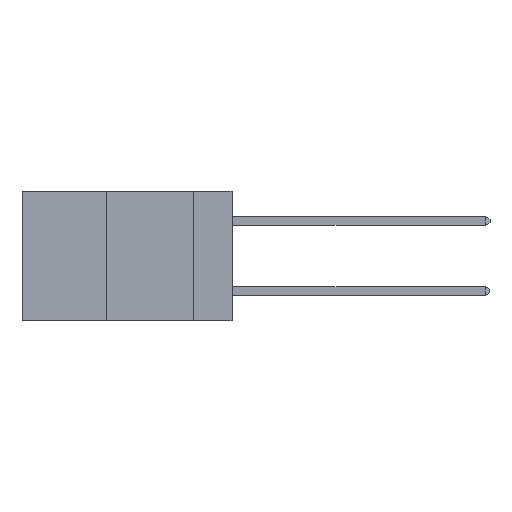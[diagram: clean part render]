
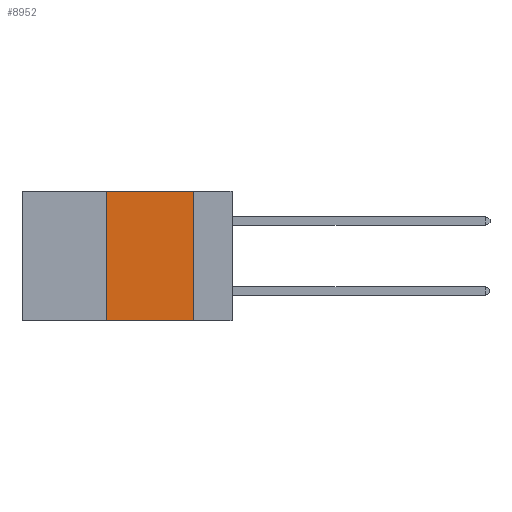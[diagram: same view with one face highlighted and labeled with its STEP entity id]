
A CAD part, left-side view. The second image highlights one B-rep face of the part: STEP entity #8952.
In plain terms, the highlighted planar face has unit normal (-1, 0, 0).
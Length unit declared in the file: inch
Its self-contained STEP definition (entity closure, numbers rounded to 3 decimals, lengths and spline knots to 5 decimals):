
#103 = LINE ( 'NONE', #3555, #1944 ) ;
#345 = ORIENTED_EDGE ( 'NONE', *, *, #6749, .T. ) ;
#522 = DIRECTION ( 'NONE',  ( 0., 0., -1. ) ) ;
#598 = LINE ( 'NONE', #9883, #2909 ) ;
#654 = VECTOR ( 'NONE', #4590, 39.37008 ) ;
#705 = CARTESIAN_POINT ( 'NONE',  ( 0., 0.6, -0.37 ) ) ;
#973 = CARTESIAN_POINT ( 'NONE',  ( 0., 0.36, -0.37 ) ) ;
#1944 = VECTOR ( 'NONE', #6691, 39.37008 ) ;
#2097 = LINE ( 'NONE', #9091, #6032 ) ;
#2643 = CARTESIAN_POINT ( 'NONE',  ( 0., 0.11, 0. ) ) ;
#2756 = PLANE ( 'NONE',  #9317 ) ;
#2809 = VERTEX_POINT ( 'NONE', #3524 ) ;
#2909 = VECTOR ( 'NONE', #5192, 39.37008 ) ;
#3524 = CARTESIAN_POINT ( 'NONE',  ( 0., 0.11, -0.37 ) ) ;
#3554 = CARTESIAN_POINT ( 'NONE',  ( 0., 0.6, 0. ) ) ;
#3555 = CARTESIAN_POINT ( 'NONE',  ( 0., 0.6, 0. ) ) ;
#3788 = ORIENTED_EDGE ( 'NONE', *, *, #3938, .F. ) ;
#3938 = EDGE_CURVE ( 'NONE', #5005, #7772, #103, .T. ) ;
#4338 = DIRECTION ( 'NONE',  ( 1., 0., 0. ) ) ;
#4590 = DIRECTION ( 'NONE',  ( 0., -1., 0. ) ) ;
#5005 = VERTEX_POINT ( 'NONE', #7924 ) ;
#5192 = DIRECTION ( 'NONE',  ( 0., 0., 1. ) ) ;
#5319 = EDGE_LOOP ( 'NONE', ( #7978, #3788, #7088, #345 ) ) ;
#5479 = FACE_OUTER_BOUND ( 'NONE', #5319, .T. ) ;
#6032 = VECTOR ( 'NONE', #522, 39.37008 ) ;
#6320 = VERTEX_POINT ( 'NONE', #973 ) ;
#6601 = EDGE_CURVE ( 'NONE', #7772, #2809, #2097, .T. ) ;
#6691 = DIRECTION ( 'NONE',  ( 0., -1., 0. ) ) ;
#6749 = EDGE_CURVE ( 'NONE', #6320, #2809, #6906, .T. ) ;
#6906 = LINE ( 'NONE', #705, #654 ) ;
#7088 = ORIENTED_EDGE ( 'NONE', *, *, #8997, .F. ) ;
#7772 = VERTEX_POINT ( 'NONE', #2643 ) ;
#7924 = CARTESIAN_POINT ( 'NONE',  ( 0., 0.36, 0. ) ) ;
#7978 = ORIENTED_EDGE ( 'NONE', *, *, #6601, .F. ) ;
#8952 = ADVANCED_FACE ( 'NONE', ( #5479 ), #2756, .F. ) ;
#8997 = EDGE_CURVE ( 'NONE', #6320, #5005, #598, .T. ) ;
#9091 = CARTESIAN_POINT ( 'NONE',  ( 0., 0.11, 0. ) ) ;
#9317 = AXIS2_PLACEMENT_3D ( 'NONE', #3554, #4338, #9811 ) ;
#9811 = DIRECTION ( 'NONE',  ( 0., 0., -1. ) ) ;
#9883 = CARTESIAN_POINT ( 'NONE',  ( 0., 0.36, 0. ) ) ;
